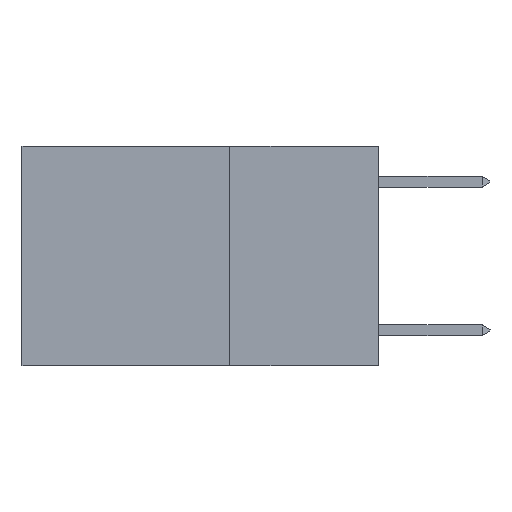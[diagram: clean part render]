
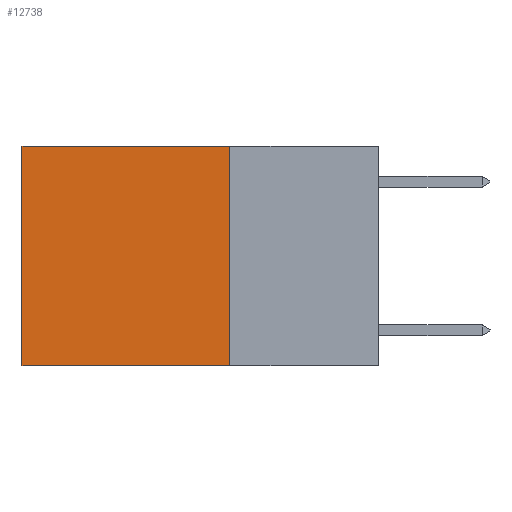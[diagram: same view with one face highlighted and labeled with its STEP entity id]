
A CAD part, left-side view. The second image highlights one B-rep face of the part: STEP entity #12738.
In plain terms, the highlighted planar face has unit normal (-1, 0, 0).
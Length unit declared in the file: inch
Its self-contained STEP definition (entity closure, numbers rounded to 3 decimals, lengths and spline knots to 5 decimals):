
#1366 = FACE_OUTER_BOUND ( 'NONE', #2986, .T. ) ;
#1538 = DIRECTION ( 'NONE',  ( 0., 1., 0. ) ) ;
#1627 = LINE ( 'NONE', #14095, #11585 ) ;
#2665 = ORIENTED_EDGE ( 'NONE', *, *, #6580, .T. ) ;
#2986 = EDGE_LOOP ( 'NONE', ( #13781, #12491, #8767, #2665 ) ) ;
#3876 = CARTESIAN_POINT ( 'NONE',  ( 0.2625, 0.6, 0. ) ) ;
#4374 = PLANE ( 'NONE',  #8994 ) ;
#4634 = CARTESIAN_POINT ( 'NONE',  ( 0.2625, 0.25, -0.37 ) ) ;
#6336 = VERTEX_POINT ( 'NONE', #3876 ) ;
#6468 = EDGE_CURVE ( 'NONE', #17470, #8220, #16102, .T. ) ;
#6580 = EDGE_CURVE ( 'NONE', #10860, #6336, #8293, .T. ) ;
#6789 = CARTESIAN_POINT ( 'NONE',  ( 0.2625, 0.25, 0. ) ) ;
#7009 = VECTOR ( 'NONE', #8492, 39.37008 ) ;
#8042 = DIRECTION ( 'NONE',  ( 0., 1., 0. ) ) ;
#8126 = CARTESIAN_POINT ( 'NONE',  ( 0.2625, 0.6, -0.37 ) ) ;
#8220 = VERTEX_POINT ( 'NONE', #8126 ) ;
#8293 = LINE ( 'NONE', #13749, #9147 ) ;
#8492 = DIRECTION ( 'NONE',  ( 0., 0., -1. ) ) ;
#8648 = DIRECTION ( 'NONE',  ( 0., 0., -1. ) ) ;
#8767 = ORIENTED_EDGE ( 'NONE', *, *, #16051, .F. ) ;
#8994 = AXIS2_PLACEMENT_3D ( 'NONE', #6789, #9789, #12127 ) ;
#9147 = VECTOR ( 'NONE', #1538, 39.37008 ) ;
#9789 = DIRECTION ( 'NONE',  ( 1., 0., 0. ) ) ;
#10860 = VERTEX_POINT ( 'NONE', #11375 ) ;
#11375 = CARTESIAN_POINT ( 'NONE',  ( 0.2625, 0.25, 0. ) ) ;
#11585 = VECTOR ( 'NONE', #8648, 39.37008 ) ;
#12127 = DIRECTION ( 'NONE',  ( 0., 0., -1. ) ) ;
#12491 = ORIENTED_EDGE ( 'NONE', *, *, #6468, .F. ) ;
#12738 = ADVANCED_FACE ( 'NONE', ( #1366 ), #4374, .F. ) ;
#13214 = CARTESIAN_POINT ( 'NONE',  ( 0.2625, 0.25, -0.37 ) ) ;
#13412 = VECTOR ( 'NONE', #8042, 39.37008 ) ;
#13749 = CARTESIAN_POINT ( 'NONE',  ( 0.2625, 0.25, 0. ) ) ;
#13781 = ORIENTED_EDGE ( 'NONE', *, *, #14234, .T. ) ;
#13846 = LINE ( 'NONE', #14112, #7009 ) ;
#14095 = CARTESIAN_POINT ( 'NONE',  ( 0.2625, 0.25, 0. ) ) ;
#14112 = CARTESIAN_POINT ( 'NONE',  ( 0.2625, 0.6, 0. ) ) ;
#14234 = EDGE_CURVE ( 'NONE', #6336, #8220, #13846, .T. ) ;
#16051 = EDGE_CURVE ( 'NONE', #10860, #17470, #1627, .T. ) ;
#16102 = LINE ( 'NONE', #13214, #13412 ) ;
#17470 = VERTEX_POINT ( 'NONE', #4634 ) ;
